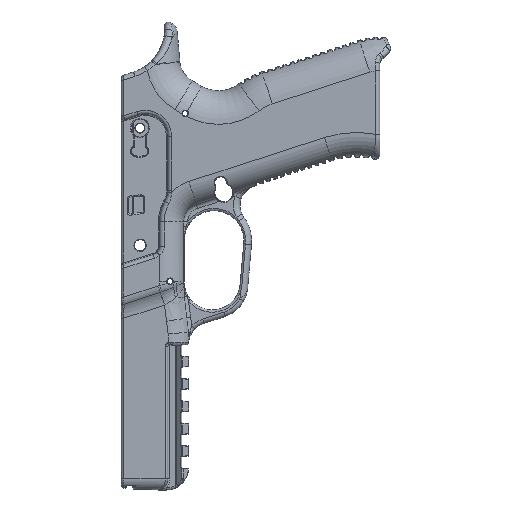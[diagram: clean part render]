
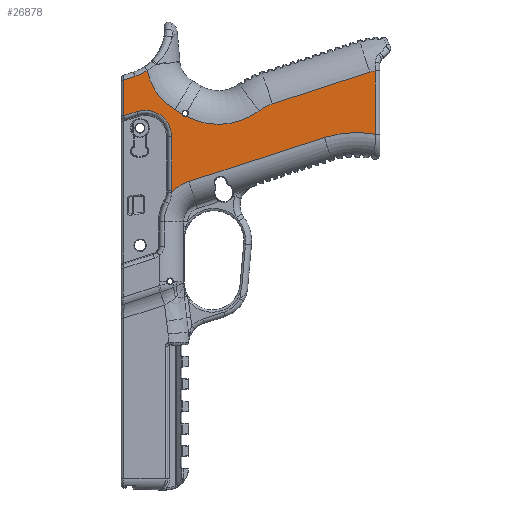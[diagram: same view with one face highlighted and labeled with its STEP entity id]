
A CAD part, left-side view. The second image highlights one B-rep face of the part: STEP entity #26878.
In plain terms, the highlighted planar face has unit normal (-1, 0, 0).
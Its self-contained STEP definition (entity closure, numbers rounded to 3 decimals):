
#758=PLANE('',#29448);
#1432=B_SPLINE_CURVE_WITH_KNOTS('',3,(#57275,#57276,#57277,#57278),
 .UNSPECIFIED.,.F.,.F.,(4,4),(0.265,0.279),
 .UNSPECIFIED.);
#1434=B_SPLINE_CURVE_WITH_KNOTS('',3,(#57299,#57300,#57301,#57302),
 .UNSPECIFIED.,.F.,.F.,(4,4),(0.191,0.207),
 .UNSPECIFIED.);
#2661=LINE('',#41577,#3895);
#2804=LINE('',#48010,#4038);
#3162=LINE('',#57314,#4396);
#3163=LINE('',#57320,#4397);
#3164=LINE('',#57322,#4398);
#3165=LINE('',#57324,#4399);
#3166=LINE('',#57328,#4400);
#3167=LINE('',#57333,#4401);
#3895=VECTOR('',#31919,10.);
#4038=VECTOR('',#32822,10.);
#4396=VECTOR('',#34968,10.);
#4397=VECTOR('',#34973,10.);
#4398=VECTOR('',#34974,10.);
#4399=VECTOR('',#34975,10.);
#4400=VECTOR('',#34978,10.);
#4401=VECTOR('',#34983,10.);
#6387=FACE_OUTER_BOUND('',#8152,.T.);
#8152=EDGE_LOOP('',(#21718,#21719,#21720,#21721,#21722,#21723,#21724,#21725,
#21726,#21727,#21728,#21729,#21730,#21731,#21732,#21733,#21734,#21735,#21736,
#21737));
#9233=CIRCLE('',#28111,20.);
#9520=CIRCLE('',#28788,46.);
#9840=CIRCLE('',#29442,1.44);
#9842=CIRCLE('',#29445,30.);
#9845=CIRCLE('',#29449,26.);
#9846=CIRCLE('',#29450,22.);
#9847=CIRCLE('',#29451,11.75);
#9848=CIRCLE('',#29452,11.75);
#9849=CIRCLE('',#29453,19.);
#9850=CIRCLE('',#29454,13.);
#10932=VERTEX_POINT('',#40484);
#10933=VERTEX_POINT('',#40486);
#10999=VERTEX_POINT('',#41576);
#11409=VERTEX_POINT('',#48007);
#11410=VERTEX_POINT('',#48009);
#11638=VERTEX_POINT('',#51732);
#12102=VERTEX_POINT('',#57110);
#12106=VERTEX_POINT('',#57148);
#12107=VERTEX_POINT('',#57150);
#12109=VERTEX_POINT('',#57219);
#12113=VERTEX_POINT('',#57313);
#12114=VERTEX_POINT('',#57315);
#12115=VERTEX_POINT('',#57317);
#12116=VERTEX_POINT('',#57319);
#12117=VERTEX_POINT('',#57321);
#12118=VERTEX_POINT('',#57323);
#12119=VERTEX_POINT('',#57325);
#12120=VERTEX_POINT('',#57327);
#12121=VERTEX_POINT('',#57329);
#12122=VERTEX_POINT('',#57332);
#13548=EDGE_CURVE('',#10932,#10933,#9233,.T.);
#13652=EDGE_CURVE('',#10933,#10999,#2661,.T.);
#14273=EDGE_CURVE('',#11409,#11410,#2804,.T.);
#14636=EDGE_CURVE('',#11638,#11409,#9520,.T.);
#15441=EDGE_CURVE('',#12106,#12107,#9840,.T.);
#15448=EDGE_CURVE('',#12109,#12106,#1432,.T.);
#15450=EDGE_CURVE('',#12107,#12102,#1434,.T.);
#15452=EDGE_CURVE('',#12102,#10932,#9842,.T.);
#15455=EDGE_CURVE('',#12113,#12109,#3162,.T.);
#15456=EDGE_CURVE('',#12114,#12113,#9845,.T.);
#15457=EDGE_CURVE('',#12115,#12114,#9846,.T.);
#15458=EDGE_CURVE('',#12116,#12115,#3163,.T.);
#15459=EDGE_CURVE('',#12117,#12116,#3164,.T.);
#15460=EDGE_CURVE('',#12118,#12117,#3165,.T.);
#15461=EDGE_CURVE('',#12119,#12118,#9847,.T.);
#15462=EDGE_CURVE('',#12120,#12119,#3166,.T.);
#15463=EDGE_CURVE('',#12121,#12120,#9848,.T.);
#15464=EDGE_CURVE('',#11410,#12121,#9849,.T.);
#15465=EDGE_CURVE('',#12122,#11638,#3167,.T.);
#15466=EDGE_CURVE('',#10999,#12122,#9850,.T.);
#21718=ORIENTED_EDGE('',*,*,#15450,.F.);
#21719=ORIENTED_EDGE('',*,*,#15441,.F.);
#21720=ORIENTED_EDGE('',*,*,#15448,.F.);
#21721=ORIENTED_EDGE('',*,*,#15455,.F.);
#21722=ORIENTED_EDGE('',*,*,#15456,.F.);
#21723=ORIENTED_EDGE('',*,*,#15457,.F.);
#21724=ORIENTED_EDGE('',*,*,#15458,.F.);
#21725=ORIENTED_EDGE('',*,*,#15459,.F.);
#21726=ORIENTED_EDGE('',*,*,#15460,.F.);
#21727=ORIENTED_EDGE('',*,*,#15461,.F.);
#21728=ORIENTED_EDGE('',*,*,#15462,.F.);
#21729=ORIENTED_EDGE('',*,*,#15463,.F.);
#21730=ORIENTED_EDGE('',*,*,#15464,.F.);
#21731=ORIENTED_EDGE('',*,*,#14273,.F.);
#21732=ORIENTED_EDGE('',*,*,#14636,.F.);
#21733=ORIENTED_EDGE('',*,*,#15465,.F.);
#21734=ORIENTED_EDGE('',*,*,#15466,.F.);
#21735=ORIENTED_EDGE('',*,*,#13652,.F.);
#21736=ORIENTED_EDGE('',*,*,#13548,.F.);
#21737=ORIENTED_EDGE('',*,*,#15452,.F.);
#26878=ADVANCED_FACE('',(#6387),#758,.F.);
#28111=AXIS2_PLACEMENT_3D('',#40487,#31771,#31772);
#28788=AXIS2_PLACEMENT_3D('',#51740,#33367,#33368);
#29442=AXIS2_PLACEMENT_3D('',#57151,#34952,#34953);
#29445=AXIS2_PLACEMENT_3D('',#57308,#34960,#34961);
#29448=AXIS2_PLACEMENT_3D('',#57312,#34966,#34967);
#29449=AXIS2_PLACEMENT_3D('',#57316,#34969,#34970);
#29450=AXIS2_PLACEMENT_3D('',#57318,#34971,#34972);
#29451=AXIS2_PLACEMENT_3D('',#57326,#34976,#34977);
#29452=AXIS2_PLACEMENT_3D('',#57330,#34979,#34980);
#29453=AXIS2_PLACEMENT_3D('',#57331,#34981,#34982);
#29454=AXIS2_PLACEMENT_3D('',#57334,#34984,#34985);
#31771=DIRECTION('center_axis',(1.,0.,0.));
#31772=DIRECTION('ref_axis',(0.,0.463,0.886));
#31919=DIRECTION('',(0.,-0.951,0.309));
#32822=DIRECTION('',(0.,0.951,-0.309));
#33367=DIRECTION('center_axis',(-1.,0.,0.));
#33368=DIRECTION('ref_axis',(0.,-0.012,1.));
#34952=DIRECTION('center_axis',(-1.,0.,0.));
#34953=DIRECTION('ref_axis',(0.,0.,-1.));
#34960=DIRECTION('center_axis',(-1.,0.,0.));
#34961=DIRECTION('ref_axis',(0.,-0.062,-0.998));
#34966=DIRECTION('center_axis',(1.,0.,0.));
#34967=DIRECTION('ref_axis',(0.,0.,-1.));
#34968=DIRECTION('',(0.,-0.866,-0.5));
#34969=DIRECTION('center_axis',(-1.,0.,0.));
#34970=DIRECTION('ref_axis',(0.,0.843,-0.537));
#34971=DIRECTION('center_axis',(-1.,0.,0.));
#34972=DIRECTION('ref_axis',(0.,-0.459,-0.889));
#34973=DIRECTION('',(0.,-0.951,0.309));
#34974=DIRECTION('',(0.,0.,1.));
#34975=DIRECTION('',(0.,0.951,-0.309));
#34976=DIRECTION('center_axis',(-1.,0.,0.));
#34977=DIRECTION('ref_axis',(0.,-0.588,0.809));
#34978=DIRECTION('',(0.,0.,1.));
#34979=DIRECTION('center_axis',(-1.,0.,0.));
#34980=DIRECTION('ref_axis',(0.,-0.968,-0.25));
#34981=DIRECTION('center_axis',(-1.,0.,0.));
#34982=DIRECTION('ref_axis',(0.,0.809,0.588));
#34983=DIRECTION('',(0.,0.,-1.));
#34984=DIRECTION('center_axis',(1.,0.,0.));
#34985=DIRECTION('ref_axis',(0.,0.129,0.992));
#40484=CARTESIAN_POINT('',(-16.,-8.989,66.499));
#40486=CARTESIAN_POINT('',(-16.,-14.885,69.578));
#40487=CARTESIAN_POINT('Origin',(-16.,-21.066,50.557));
#41576=CARTESIAN_POINT('',(-16.,-58.483,83.744));
#41577=CARTESIAN_POINT('',(-16.,-1.581,65.256));
#48007=CARTESIAN_POINT('',(-16.,-38.199,54.547));
#48009=CARTESIAN_POINT('',(-16.,22.371,34.867));
#48010=CARTESIAN_POINT('',(-16.,-16.559,47.516));
#51732=CARTESIAN_POINT('',(-16.,-61.,55.99));
#51740=CARTESIAN_POINT('Origin',(-16.,-52.414,10.798));
#57110=CARTESIAN_POINT('',(-16.,23.415,64.033));
#57148=CARTESIAN_POINT('',(-16.,25.401,65.017));
#57150=CARTESIAN_POINT('',(-16.,23.579,63.972));
#57151=CARTESIAN_POINT('Origin',(-16.,24.,65.349));
#57219=CARTESIAN_POINT('',(-16.,25.431,65.184));
#57275=CARTESIAN_POINT('Ctrl Pts',(-16.,25.431,65.184));
#57276=CARTESIAN_POINT('Ctrl Pts',(-16.,25.424,65.127));
#57277=CARTESIAN_POINT('Ctrl Pts',(-16.,25.414,65.071));
#57278=CARTESIAN_POINT('Ctrl Pts',(-16.,25.401,65.017));
#57299=CARTESIAN_POINT('Ctrl Pts',(-16.,23.579,63.972));
#57300=CARTESIAN_POINT('Ctrl Pts',(-16.,23.523,63.989));
#57301=CARTESIAN_POINT('Ctrl Pts',(-16.,23.468,64.009));
#57302=CARTESIAN_POINT('Ctrl Pts',(-16.,23.415,64.033));
#57308=CARTESIAN_POINT('Origin',(-16.,9.127,90.412));
#57312=CARTESIAN_POINT('Origin',(-16.,-7.789,0.877));
#57313=CARTESIAN_POINT('',(-16.,28.457,66.931));
#57314=CARTESIAN_POINT('',(-16.,0.564,50.827));
#57315=CARTESIAN_POINT('',(-16.,40.986,84.52));
#57316=CARTESIAN_POINT('Origin',(-16.,15.457,89.448));
#57317=CARTESIAN_POINT('',(-16.,46.448,81.863));
#57318=CARTESIAN_POINT('Origin',(-16.,53.246,102.787));
#57319=CARTESIAN_POINT('',(-16.,51.5,80.222));
#57320=CARTESIAN_POINT('',(-16.,36.537,85.084));
#57321=CARTESIAN_POINT('',(-16.,51.5,64.187));
#57322=CARTESIAN_POINT('',(-16.,51.5,-51.061));
#57323=CARTESIAN_POINT('',(-16.,45.502,66.136));
#57324=CARTESIAN_POINT('',(-16.,34.76,69.626));
#57325=CARTESIAN_POINT('',(-16.,30.121,54.961));
#57326=CARTESIAN_POINT('Origin',(-16.,41.871,54.961));
#57327=CARTESIAN_POINT('',(-16.,30.121,30.843));
#57328=CARTESIAN_POINT('',(-16.,30.121,27.919));
#57329=CARTESIAN_POINT('',(-16.,30.151,30.012));
#57330=CARTESIAN_POINT('Origin',(-16.,41.871,30.843));
#57331=CARTESIAN_POINT('Origin',(-16.,16.5,16.797));
#57332=CARTESIAN_POINT('',(-16.,-61.,84.294));
#57333=CARTESIAN_POINT('',(-16.,-61.,44.851));
#57334=CARTESIAN_POINT('Origin',(-16.,-62.5,71.38));
